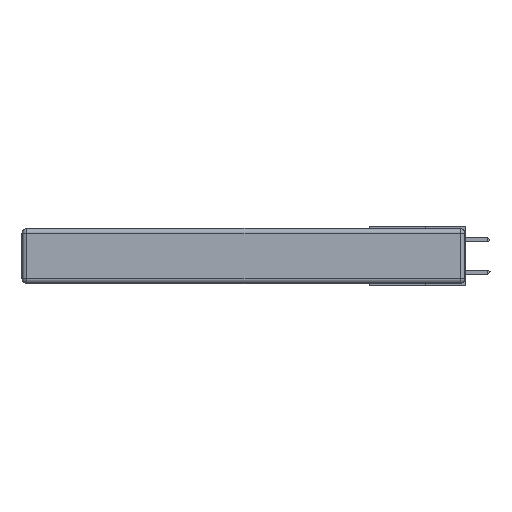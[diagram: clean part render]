
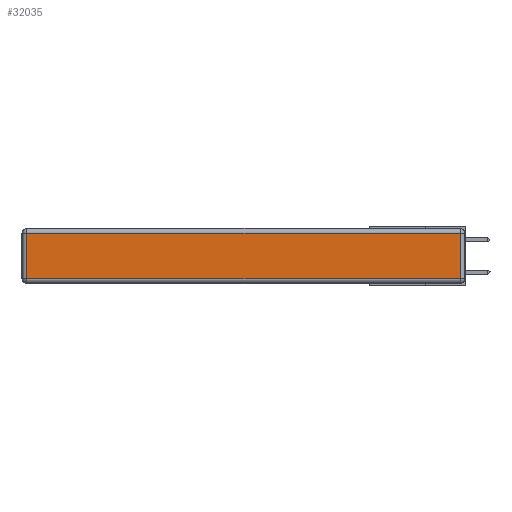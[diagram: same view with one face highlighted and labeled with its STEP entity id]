
A CAD part, left-side view. The second image highlights one B-rep face of the part: STEP entity #32035.
In plain terms, the highlighted planar face has unit normal (-1, 0, 0).
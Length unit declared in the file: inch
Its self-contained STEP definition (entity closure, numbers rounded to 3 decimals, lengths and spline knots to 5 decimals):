
#1861 = EDGE_CURVE ( 'NONE', #31766, #12041, #26984, .T. ) ;
#1991 = CARTESIAN_POINT ( 'NONE',  ( 0., 2.72, -0.03 ) ) ;
#3834 = DIRECTION ( 'NONE',  ( 0., -1., 0. ) ) ;
#4830 = DIRECTION ( 'NONE',  ( 0., 0., 1. ) ) ;
#5324 = LINE ( 'NONE', #32675, #31624 ) ;
#6323 = FACE_OUTER_BOUND ( 'NONE', #15179, .T. ) ;
#6548 = DIRECTION ( 'NONE',  ( 0., 0., -1. ) ) ;
#6778 = LINE ( 'NONE', #30681, #12849 ) ;
#7627 = DIRECTION ( 'NONE',  ( -1., 0., 0. ) ) ;
#9889 = CARTESIAN_POINT ( 'NONE',  ( 0., 0., -0.343 ) ) ;
#12041 = VERTEX_POINT ( 'NONE', #27997 ) ;
#12849 = VECTOR ( 'NONE', #28515, 39.37008 ) ;
#13608 = VECTOR ( 'NONE', #6548, 39.37008 ) ;
#14821 = CARTESIAN_POINT ( 'NONE',  ( 0., 2.72, -0.343 ) ) ;
#15179 = EDGE_LOOP ( 'NONE', ( #17718, #28467, #16890, #27827 ) ) ;
#16611 = CARTESIAN_POINT ( 'NONE',  ( 0., 0., -0.313 ) ) ;
#16890 = ORIENTED_EDGE ( 'NONE', *, *, #25320, .T. ) ;
#17718 = ORIENTED_EDGE ( 'NONE', *, *, #1861, .T. ) ;
#20142 = VERTEX_POINT ( 'NONE', #1991 ) ;
#21696 = LINE ( 'NONE', #14821, #13608 ) ;
#24231 = VERTEX_POINT ( 'NONE', #27861 ) ;
#25320 = EDGE_CURVE ( 'NONE', #24231, #20142, #6778, .T. ) ;
#26357 = EDGE_CURVE ( 'NONE', #20142, #31766, #21696, .T. ) ;
#26818 = CARTESIAN_POINT ( 'NONE',  ( 0., 2.72, -0.313 ) ) ;
#26984 = LINE ( 'NONE', #16611, #30204 ) ;
#27103 = AXIS2_PLACEMENT_3D ( 'NONE', #9889, #7627, #4830 ) ;
#27827 = ORIENTED_EDGE ( 'NONE', *, *, #26357, .T. ) ;
#27861 = CARTESIAN_POINT ( 'NONE',  ( 0., 0.03, -0.03 ) ) ;
#27997 = CARTESIAN_POINT ( 'NONE',  ( 0., 0.03, -0.313 ) ) ;
#28467 = ORIENTED_EDGE ( 'NONE', *, *, #28486, .T. ) ;
#28486 = EDGE_CURVE ( 'NONE', #12041, #24231, #5324, .T. ) ;
#28515 = DIRECTION ( 'NONE',  ( 0., 1., 0. ) ) ;
#30204 = VECTOR ( 'NONE', #3834, 39.37008 ) ;
#30681 = CARTESIAN_POINT ( 'NONE',  ( 0., 2.75, -0.03 ) ) ;
#30817 = PLANE ( 'NONE',  #27103 ) ;
#31624 = VECTOR ( 'NONE', #32566, 39.37008 ) ;
#31766 = VERTEX_POINT ( 'NONE', #26818 ) ;
#32035 = ADVANCED_FACE ( 'NONE', ( #6323 ), #30817, .T. ) ;
#32566 = DIRECTION ( 'NONE',  ( 0., 0., 1. ) ) ;
#32675 = CARTESIAN_POINT ( 'NONE',  ( 0., 0.03, -0.343 ) ) ;
